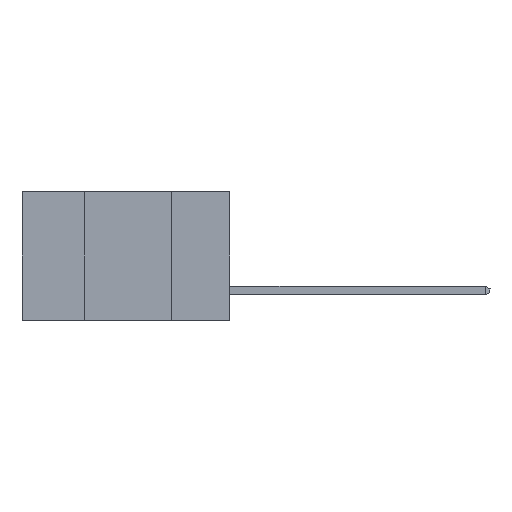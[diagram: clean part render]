
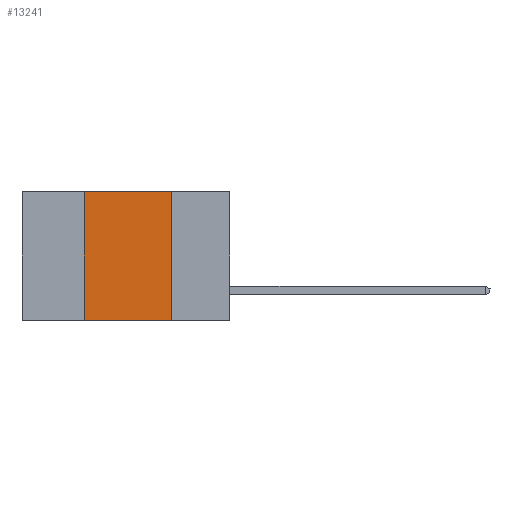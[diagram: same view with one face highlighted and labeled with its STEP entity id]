
A CAD part, left-side view. The second image highlights one B-rep face of the part: STEP entity #13241.
In plain terms, the highlighted planar face has unit normal (-1, 0, 0).
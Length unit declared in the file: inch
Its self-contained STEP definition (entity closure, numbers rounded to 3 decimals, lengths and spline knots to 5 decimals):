
#508 = VECTOR ( 'NONE', #5179, 39.37008 ) ;
#2521 = EDGE_CURVE ( 'NONE', #5663, #8470, #17036, .T. ) ;
#3118 = DIRECTION ( 'NONE',  ( 0., -1., 0. ) ) ;
#3148 = CARTESIAN_POINT ( 'NONE',  ( 0., 0.6, 0. ) ) ;
#4726 = LINE ( 'NONE', #17702, #7685 ) ;
#5073 = LINE ( 'NONE', #18166, #508 ) ;
#5179 = DIRECTION ( 'NONE',  ( 0., -1., 0. ) ) ;
#5663 = VERTEX_POINT ( 'NONE', #10091 ) ;
#6027 = DIRECTION ( 'NONE',  ( 1., 0., 0. ) ) ;
#7061 = VERTEX_POINT ( 'NONE', #19730 ) ;
#7348 = CARTESIAN_POINT ( 'NONE',  ( 0., 0.42, -0.37 ) ) ;
#7685 = VECTOR ( 'NONE', #3118, 39.37008 ) ;
#7846 = PLANE ( 'NONE',  #8331 ) ;
#8331 = AXIS2_PLACEMENT_3D ( 'NONE', #3148, #6027, #19216 ) ;
#8370 = EDGE_LOOP ( 'NONE', ( #9388, #12072, #17916, #17479 ) ) ;
#8470 = VERTEX_POINT ( 'NONE', #17495 ) ;
#9388 = ORIENTED_EDGE ( 'NONE', *, *, #15760, .F. ) ;
#10091 = CARTESIAN_POINT ( 'NONE',  ( 0., 0.42, -0.37 ) ) ;
#11587 = EDGE_CURVE ( 'NONE', #5663, #16146, #5073, .T. ) ;
#11996 = EDGE_CURVE ( 'NONE', #8470, #7061, #4726, .T. ) ;
#12072 = ORIENTED_EDGE ( 'NONE', *, *, #11996, .F. ) ;
#12885 = CARTESIAN_POINT ( 'NONE',  ( 0., 0.17, -0.37 ) ) ;
#13241 = ADVANCED_FACE ( 'NONE', ( #20816 ), #7846, .F. ) ;
#15760 = EDGE_CURVE ( 'NONE', #7061, #16146, #19390, .T. ) ;
#16098 = DIRECTION ( 'NONE',  ( 0., 0., -1. ) ) ;
#16146 = VERTEX_POINT ( 'NONE', #12885 ) ;
#17036 = LINE ( 'NONE', #7348, #18856 ) ;
#17479 = ORIENTED_EDGE ( 'NONE', *, *, #11587, .T. ) ;
#17495 = CARTESIAN_POINT ( 'NONE',  ( 0., 0.42, 0. ) ) ;
#17689 = CARTESIAN_POINT ( 'NONE',  ( 0., 0.17, -0.37 ) ) ;
#17702 = CARTESIAN_POINT ( 'NONE',  ( 0., 0.6, 0. ) ) ;
#17916 = ORIENTED_EDGE ( 'NONE', *, *, #2521, .F. ) ;
#18166 = CARTESIAN_POINT ( 'NONE',  ( 0., 0.6, -0.37 ) ) ;
#18856 = VECTOR ( 'NONE', #20318, 39.37008 ) ;
#18950 = VECTOR ( 'NONE', #16098, 39.37008 ) ;
#19216 = DIRECTION ( 'NONE',  ( 0., 0., -1. ) ) ;
#19390 = LINE ( 'NONE', #17689, #18950 ) ;
#19730 = CARTESIAN_POINT ( 'NONE',  ( 0., 0.17, 0. ) ) ;
#20318 = DIRECTION ( 'NONE',  ( 0., 0., 1. ) ) ;
#20816 = FACE_OUTER_BOUND ( 'NONE', #8370, .T. ) ;
